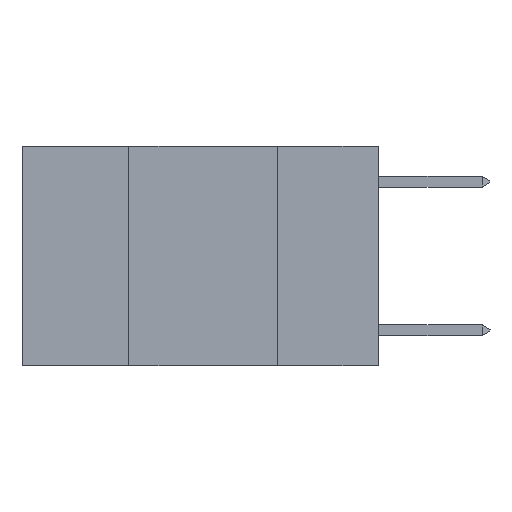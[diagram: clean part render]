
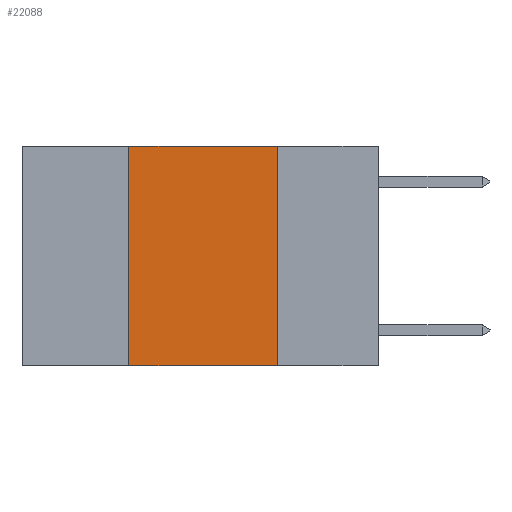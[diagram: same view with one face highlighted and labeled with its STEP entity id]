
A CAD part, left-side view. The second image highlights one B-rep face of the part: STEP entity #22088.
In plain terms, the highlighted planar face has unit normal (-1, 0, 0).
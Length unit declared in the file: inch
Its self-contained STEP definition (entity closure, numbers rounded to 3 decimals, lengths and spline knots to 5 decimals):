
#799 = EDGE_CURVE ( 'NONE', #1653, #5487, #19719, .T. ) ;
#1418 = EDGE_CURVE ( 'NONE', #5340, #1653, #14648, .T. ) ;
#1653 = VERTEX_POINT ( 'NONE', #8113 ) ;
#2455 = LINE ( 'NONE', #9796, #13862 ) ;
#3040 = DIRECTION ( 'NONE',  ( 1., 0., 0. ) ) ;
#5083 = LINE ( 'NONE', #9558, #17128 ) ;
#5340 = VERTEX_POINT ( 'NONE', #28644 ) ;
#5487 = VERTEX_POINT ( 'NONE', #13414 ) ;
#5954 = DIRECTION ( 'NONE',  ( 0., -1., 0. ) ) ;
#8113 = CARTESIAN_POINT ( 'NONE',  ( 0., 0.42, 0. ) ) ;
#9558 = CARTESIAN_POINT ( 'NONE',  ( 0., 0.17, 0. ) ) ;
#9791 = CARTESIAN_POINT ( 'NONE',  ( 0., 0.6, 0. ) ) ;
#9796 = CARTESIAN_POINT ( 'NONE',  ( 0., 0.6, -0.37 ) ) ;
#10919 = CARTESIAN_POINT ( 'NONE',  ( 0., 0.17, -0.37 ) ) ;
#13135 = EDGE_LOOP ( 'NONE', ( #25706, #26063, #26185, #27076 ) ) ;
#13414 = CARTESIAN_POINT ( 'NONE',  ( 0., 0.17, 0. ) ) ;
#13862 = VECTOR ( 'NONE', #18920, 39.37008 ) ;
#14648 = LINE ( 'NONE', #21784, #15226 ) ;
#14695 = EDGE_CURVE ( 'NONE', #5340, #25460, #2455, .T. ) ;
#15226 = VECTOR ( 'NONE', #16733, 39.37008 ) ;
#16620 = PLANE ( 'NONE',  #17577 ) ;
#16733 = DIRECTION ( 'NONE',  ( 0., 0., 1. ) ) ;
#17128 = VECTOR ( 'NONE', #25467, 39.37008 ) ;
#17577 = AXIS2_PLACEMENT_3D ( 'NONE', #9791, #3040, #18917 ) ;
#18784 = CARTESIAN_POINT ( 'NONE',  ( 0., 0.6, 0. ) ) ;
#18917 = DIRECTION ( 'NONE',  ( 0., 0., -1. ) ) ;
#18920 = DIRECTION ( 'NONE',  ( 0., -1., 0. ) ) ;
#19719 = LINE ( 'NONE', #18784, #19813 ) ;
#19813 = VECTOR ( 'NONE', #5954, 39.37008 ) ;
#21521 = FACE_OUTER_BOUND ( 'NONE', #13135, .T. ) ;
#21784 = CARTESIAN_POINT ( 'NONE',  ( 0., 0.42, 0. ) ) ;
#22088 = ADVANCED_FACE ( 'NONE', ( #21521 ), #16620, .F. ) ;
#24996 = EDGE_CURVE ( 'NONE', #5487, #25460, #5083, .T. ) ;
#25460 = VERTEX_POINT ( 'NONE', #10919 ) ;
#25467 = DIRECTION ( 'NONE',  ( 0., 0., -1. ) ) ;
#25706 = ORIENTED_EDGE ( 'NONE', *, *, #24996, .F. ) ;
#26063 = ORIENTED_EDGE ( 'NONE', *, *, #799, .F. ) ;
#26185 = ORIENTED_EDGE ( 'NONE', *, *, #1418, .F. ) ;
#27076 = ORIENTED_EDGE ( 'NONE', *, *, #14695, .T. ) ;
#28644 = CARTESIAN_POINT ( 'NONE',  ( 0., 0.42, -0.37 ) ) ;
